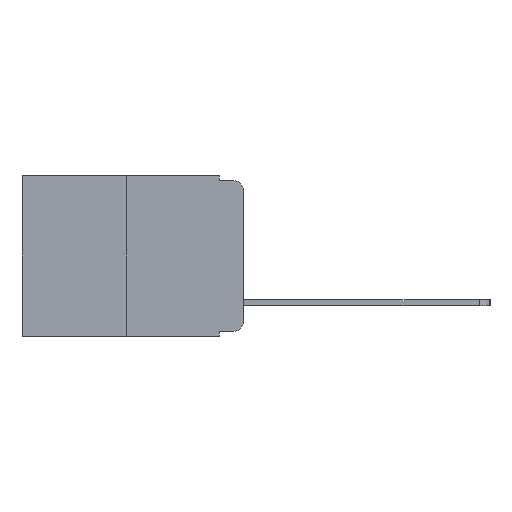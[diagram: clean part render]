
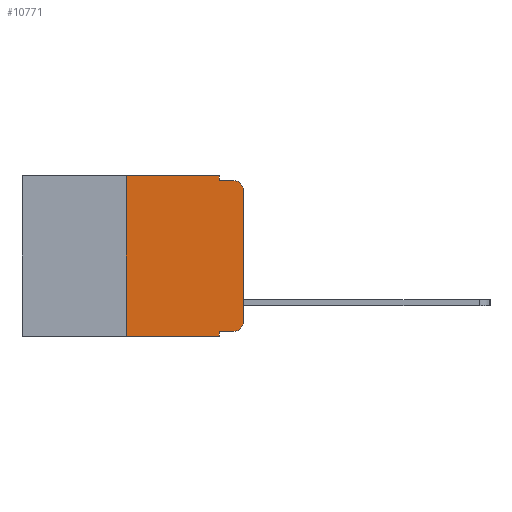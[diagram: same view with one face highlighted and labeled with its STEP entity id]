
A CAD part, left-side view. The second image highlights one B-rep face of the part: STEP entity #10771.
In plain terms, the highlighted planar face has unit normal (-1, 0, 0).
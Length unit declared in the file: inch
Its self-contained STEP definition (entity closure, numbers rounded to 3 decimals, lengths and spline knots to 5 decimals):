
#50 = EDGE_CURVE ( 'NONE', #2653, #2351, #6041, .T. ) ;
#66 = CARTESIAN_POINT ( 'NONE',  ( 0., 0.02, -0.333 ) ) ;
#70 = DIRECTION ( 'NONE',  ( -1., 0., 0. ) ) ;
#289 = VERTEX_POINT ( 'NONE', #11126 ) ;
#309 = VECTOR ( 'NONE', #9468, 39.37008 ) ;
#319 = DIRECTION ( 'NONE',  ( -1., 0., 0. ) ) ;
#372 = ORIENTED_EDGE ( 'NONE', *, *, #433, .T. ) ;
#428 = CARTESIAN_POINT ( 'NONE',  ( 0., 0., 0. ) ) ;
#433 = EDGE_CURVE ( 'NONE', #3203, #11966, #6925, .T. ) ;
#491 = CARTESIAN_POINT ( 'NONE',  ( 0., 0.051, -0.01 ) ) ;
#1177 = EDGE_CURVE ( 'NONE', #5297, #289, #6454, .T. ) ;
#1319 = VECTOR ( 'NONE', #11149, 39.37008 ) ;
#1581 = VERTEX_POINT ( 'NONE', #7826 ) ;
#1796 = VECTOR ( 'NONE', #2921, 39.37008 ) ;
#1803 = ORIENTED_EDGE ( 'NONE', *, *, #7417, .T. ) ;
#1968 = DIRECTION ( 'NONE',  ( 0., 0., -1. ) ) ;
#2035 = DIRECTION ( 'NONE',  ( 0., -1., 0. ) ) ;
#2215 = ORIENTED_EDGE ( 'NONE', *, *, #5276, .F. ) ;
#2260 = CARTESIAN_POINT ( 'NONE',  ( 0., 0.051, 0. ) ) ;
#2351 = VERTEX_POINT ( 'NONE', #6722 ) ;
#2401 = EDGE_CURVE ( 'NONE', #11966, #2351, #3295, .T. ) ;
#2438 = CARTESIAN_POINT ( 'NONE',  ( 0., 0.25, 0. ) ) ;
#2653 = VERTEX_POINT ( 'NONE', #491 ) ;
#2659 = EDGE_CURVE ( 'NONE', #10111, #5297, #8238, .T. ) ;
#2900 = LINE ( 'NONE', #3723, #309 ) ;
#2921 = DIRECTION ( 'NONE',  ( 0., 0., 1. ) ) ;
#3055 = FACE_OUTER_BOUND ( 'NONE', #11919, .T. ) ;
#3203 = VERTEX_POINT ( 'NONE', #8046 ) ;
#3295 = CIRCLE ( 'NONE', #3343, 0.02 ) ;
#3343 = AXIS2_PLACEMENT_3D ( 'NONE', #5886, #70, #6842 ) ;
#3433 = DIRECTION ( 'NONE',  ( 0., 0., 1. ) ) ;
#3654 = CARTESIAN_POINT ( 'NONE',  ( 0., 0.25, -0.343 ) ) ;
#3703 = LINE ( 'NONE', #12103, #11051 ) ;
#3723 = CARTESIAN_POINT ( 'NONE',  ( 0., 0.051, 0. ) ) ;
#3729 = LINE ( 'NONE', #2260, #8539 ) ;
#4237 = AXIS2_PLACEMENT_3D ( 'NONE', #6773, #7722, #1968 ) ;
#5009 = PLANE ( 'NONE',  #4237 ) ;
#5276 = EDGE_CURVE ( 'NONE', #8498, #1581, #2900, .T. ) ;
#5297 = VERTEX_POINT ( 'NONE', #7595 ) ;
#5431 = EDGE_CURVE ( 'NONE', #10111, #1581, #10998, .T. ) ;
#5886 = CARTESIAN_POINT ( 'NONE',  ( 0., 0.02, -0.03 ) ) ;
#6041 = LINE ( 'NONE', #10789, #8877 ) ;
#6134 = CARTESIAN_POINT ( 'NONE',  ( 0., 0.02, -0.313 ) ) ;
#6279 = AXIS2_PLACEMENT_3D ( 'NONE', #6134, #319, #7092 ) ;
#6454 = LINE ( 'NONE', #9131, #1319 ) ;
#6722 = CARTESIAN_POINT ( 'NONE',  ( 0., 0.02, -0.01 ) ) ;
#6773 = CARTESIAN_POINT ( 'NONE',  ( 0., 0.473, 0. ) ) ;
#6842 = DIRECTION ( 'NONE',  ( 0., 0., -1. ) ) ;
#6887 = DIRECTION ( 'NONE',  ( 0., -1., 0. ) ) ;
#6900 = ORIENTED_EDGE ( 'NONE', *, *, #2401, .T. ) ;
#6925 = LINE ( 'NONE', #428, #1796 ) ;
#7092 = DIRECTION ( 'NONE',  ( 0., 0., -1. ) ) ;
#7263 = VERTEX_POINT ( 'NONE', #66 ) ;
#7417 = EDGE_CURVE ( 'NONE', #7263, #3203, #8122, .T. ) ;
#7595 = CARTESIAN_POINT ( 'NONE',  ( 0., 0.25, 0. ) ) ;
#7722 = DIRECTION ( 'NONE',  ( 1., 0., 0. ) ) ;
#7798 = CARTESIAN_POINT ( 'NONE',  ( 0., 0.473, -0.343 ) ) ;
#7826 = CARTESIAN_POINT ( 'NONE',  ( 0., 0.051, -0.343 ) ) ;
#7966 = ORIENTED_EDGE ( 'NONE', *, *, #9337, .T. ) ;
#8046 = CARTESIAN_POINT ( 'NONE',  ( 0., 0., -0.313 ) ) ;
#8082 = CARTESIAN_POINT ( 'NONE',  ( 0., 0.051, -0.333 ) ) ;
#8105 = ORIENTED_EDGE ( 'NONE', *, *, #50, .F. ) ;
#8122 = CIRCLE ( 'NONE', #6279, 0.02 ) ;
#8238 = LINE ( 'NONE', #2438, #10492 ) ;
#8459 = VECTOR ( 'NONE', #2035, 39.37008 ) ;
#8462 = EDGE_CURVE ( 'NONE', #289, #2653, #3729, .T. ) ;
#8498 = VERTEX_POINT ( 'NONE', #8082 ) ;
#8539 = VECTOR ( 'NONE', #9956, 39.37008 ) ;
#8780 = ORIENTED_EDGE ( 'NONE', *, *, #5431, .T. ) ;
#8877 = VECTOR ( 'NONE', #6887, 39.37008 ) ;
#9131 = CARTESIAN_POINT ( 'NONE',  ( 0., 0.473, 0. ) ) ;
#9255 = DIRECTION ( 'NONE',  ( 0., -1., 0. ) ) ;
#9337 = EDGE_CURVE ( 'NONE', #8498, #7263, #3703, .T. ) ;
#9468 = DIRECTION ( 'NONE',  ( 0., 0., -1. ) ) ;
#9538 = CARTESIAN_POINT ( 'NONE',  ( 0., 0., -0.03 ) ) ;
#9761 = ORIENTED_EDGE ( 'NONE', *, *, #1177, .F. ) ;
#9956 = DIRECTION ( 'NONE',  ( 0., 0., -1. ) ) ;
#10111 = VERTEX_POINT ( 'NONE', #3654 ) ;
#10423 = ORIENTED_EDGE ( 'NONE', *, *, #2659, .F. ) ;
#10492 = VECTOR ( 'NONE', #3433, 39.37008 ) ;
#10771 = ADVANCED_FACE ( 'NONE', ( #3055 ), #5009, .F. ) ;
#10789 = CARTESIAN_POINT ( 'NONE',  ( 0., 0.051, -0.01 ) ) ;
#10998 = LINE ( 'NONE', #7798, #8459 ) ;
#11051 = VECTOR ( 'NONE', #9255, 39.37008 ) ;
#11126 = CARTESIAN_POINT ( 'NONE',  ( 0., 0.051, 0. ) ) ;
#11149 = DIRECTION ( 'NONE',  ( 0., -1., 0. ) ) ;
#11398 = ORIENTED_EDGE ( 'NONE', *, *, #8462, .F. ) ;
#11919 = EDGE_LOOP ( 'NONE', ( #372, #6900, #8105, #11398, #9761, #10423, #8780, #2215, #7966, #1803 ) ) ;
#11966 = VERTEX_POINT ( 'NONE', #9538 ) ;
#12103 = CARTESIAN_POINT ( 'NONE',  ( 0., 0.051, -0.333 ) ) ;
